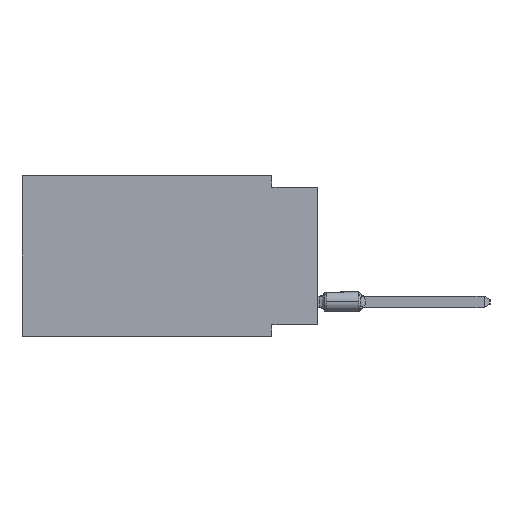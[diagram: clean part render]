
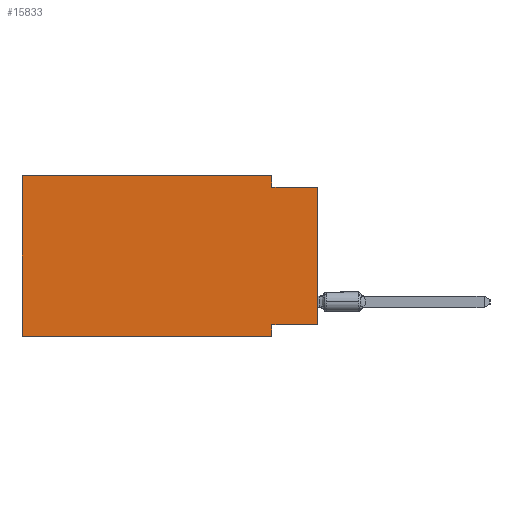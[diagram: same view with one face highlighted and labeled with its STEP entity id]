
A CAD part, left-side view. The second image highlights one B-rep face of the part: STEP entity #15833.
In plain terms, the highlighted planar face has unit normal (-1, 0, 0).
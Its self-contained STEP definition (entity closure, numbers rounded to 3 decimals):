
#2343 = DIRECTION ( 'NONE',  ( 1., 0., 0. ) ) ;
#2830 = CARTESIAN_POINT ( 'NONE',  ( 0., 0., -0.635 ) ) ;
#3074 = DIRECTION ( 'NONE',  ( 0., 0., -1. ) ) ;
#3347 = VERTEX_POINT ( 'NONE', #22993 ) ;
#3587 = CARTESIAN_POINT ( 'NONE',  ( 0., 0., 0. ) ) ;
#4840 = VECTOR ( 'NONE', #38011, 1000. ) ;
#5875 = VERTEX_POINT ( 'NONE', #41735 ) ;
#6021 = VECTOR ( 'NONE', #34239, 1000. ) ;
#7030 = VECTOR ( 'NONE', #20610, 1000. ) ;
#9397 = VERTEX_POINT ( 'NONE', #32494 ) ;
#10653 = EDGE_CURVE ( 'NONE', #36518, #14040, #44308, .T. ) ;
#10917 = LINE ( 'NONE', #43354, #23785 ) ;
#11809 = CARTESIAN_POINT ( 'NONE',  ( 0., 0., -0.635 ) ) ;
#13219 = CARTESIAN_POINT ( 'NONE',  ( 0., 16.383, -8.89 ) ) ;
#14040 = VERTEX_POINT ( 'NONE', #32887 ) ;
#15454 = EDGE_CURVE ( 'NONE', #36518, #19072, #39714, .T. ) ;
#15596 = ORIENTED_EDGE ( 'NONE', *, *, #10653, .F. ) ;
#15833 = ADVANCED_FACE ( 'NONE', ( #25839 ), #49849, .F. ) ;
#15977 = VECTOR ( 'NONE', #40023, 1000. ) ;
#16514 = ORIENTED_EDGE ( 'NONE', *, *, #48632, .F. ) ;
#17523 = CARTESIAN_POINT ( 'NONE',  ( 0., 2.54, -8.89 ) ) ;
#17560 = VERTEX_POINT ( 'NONE', #17523 ) ;
#19072 = VERTEX_POINT ( 'NONE', #2830 ) ;
#19172 = EDGE_CURVE ( 'NONE', #3347, #30265, #23130, .T. ) ;
#19668 = DIRECTION ( 'NONE',  ( 0., 0., 1. ) ) ;
#20309 = CARTESIAN_POINT ( 'NONE',  ( 0., 0., -8.255 ) ) ;
#20610 = DIRECTION ( 'NONE',  ( 0., 0., 1. ) ) ;
#22993 = CARTESIAN_POINT ( 'NONE',  ( 0., 2.54, 0. ) ) ;
#23130 = LINE ( 'NONE', #39205, #38003 ) ;
#23785 = VECTOR ( 'NONE', #51530, 1000. ) ;
#24818 = EDGE_CURVE ( 'NONE', #5875, #3347, #10917, .T. ) ;
#25150 = CARTESIAN_POINT ( 'NONE',  ( 0., 0., -8.255 ) ) ;
#25839 = FACE_OUTER_BOUND ( 'NONE', #42997, .T. ) ;
#26076 = CARTESIAN_POINT ( 'NONE',  ( 0., 2.54, -8.89 ) ) ;
#26350 = LINE ( 'NONE', #11809, #15977 ) ;
#26601 = EDGE_CURVE ( 'NONE', #30265, #19072, #26350, .T. ) ;
#29179 = VECTOR ( 'NONE', #36395, 1000. ) ;
#29244 = ORIENTED_EDGE ( 'NONE', *, *, #15454, .T. ) ;
#29557 = DIRECTION ( 'NONE',  ( 0., 0., -1. ) ) ;
#29822 = CARTESIAN_POINT ( 'NONE',  ( 0., 16.383, 0. ) ) ;
#29893 = ORIENTED_EDGE ( 'NONE', *, *, #19172, .F. ) ;
#30012 = ORIENTED_EDGE ( 'NONE', *, *, #24818, .F. ) ;
#30265 = VERTEX_POINT ( 'NONE', #34369 ) ;
#31331 = EDGE_CURVE ( 'NONE', #9397, #17560, #49093, .T. ) ;
#32494 = CARTESIAN_POINT ( 'NONE',  ( 0., 16.383, -8.89 ) ) ;
#32887 = CARTESIAN_POINT ( 'NONE',  ( 0., 2.54, -8.255 ) ) ;
#33528 = CARTESIAN_POINT ( 'NONE',  ( 0., 16.383, 0. ) ) ;
#34239 = DIRECTION ( 'NONE',  ( 0., 0., -1. ) ) ;
#34369 = CARTESIAN_POINT ( 'NONE',  ( 0., 2.54, -0.635 ) ) ;
#34495 = EDGE_CURVE ( 'NONE', #9397, #5875, #41715, .T. ) ;
#36270 = ORIENTED_EDGE ( 'NONE', *, *, #31331, .T. ) ;
#36395 = DIRECTION ( 'NONE',  ( 0., 1., 0. ) ) ;
#36518 = VERTEX_POINT ( 'NONE', #25150 ) ;
#38003 = VECTOR ( 'NONE', #3074, 1000. ) ;
#38011 = DIRECTION ( 'NONE',  ( 0., -1., 0. ) ) ;
#38175 = ORIENTED_EDGE ( 'NONE', *, *, #34495, .F. ) ;
#39205 = CARTESIAN_POINT ( 'NONE',  ( 0., 2.54, 0. ) ) ;
#39714 = LINE ( 'NONE', #3587, #47129 ) ;
#40023 = DIRECTION ( 'NONE',  ( 0., -1., 0. ) ) ;
#40393 = AXIS2_PLACEMENT_3D ( 'NONE', #29822, #2343, #29557 ) ;
#41715 = LINE ( 'NONE', #33528, #7030 ) ;
#41735 = CARTESIAN_POINT ( 'NONE',  ( 0., 16.383, 0. ) ) ;
#42934 = LINE ( 'NONE', #26076, #6021 ) ;
#42997 = EDGE_LOOP ( 'NONE', ( #29244, #43969, #29893, #30012, #38175, #36270, #16514, #15596 ) ) ;
#43354 = CARTESIAN_POINT ( 'NONE',  ( 0., 16.383, 0. ) ) ;
#43969 = ORIENTED_EDGE ( 'NONE', *, *, #26601, .F. ) ;
#44308 = LINE ( 'NONE', #20309, #29179 ) ;
#47129 = VECTOR ( 'NONE', #19668, 1000. ) ;
#48632 = EDGE_CURVE ( 'NONE', #14040, #17560, #42934, .T. ) ;
#49093 = LINE ( 'NONE', #13219, #4840 ) ;
#49849 = PLANE ( 'NONE',  #40393 ) ;
#51530 = DIRECTION ( 'NONE',  ( 0., -1., 0. ) ) ;
